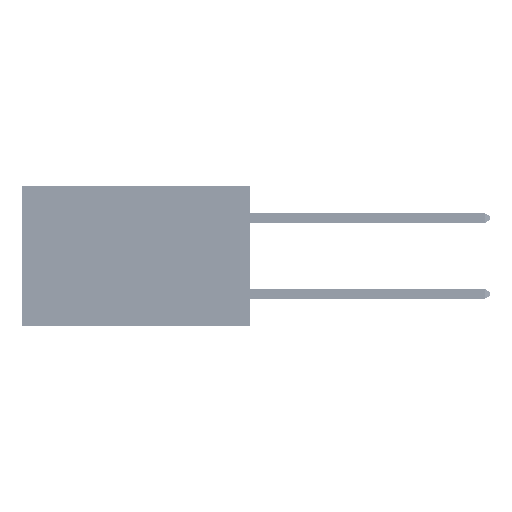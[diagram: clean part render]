
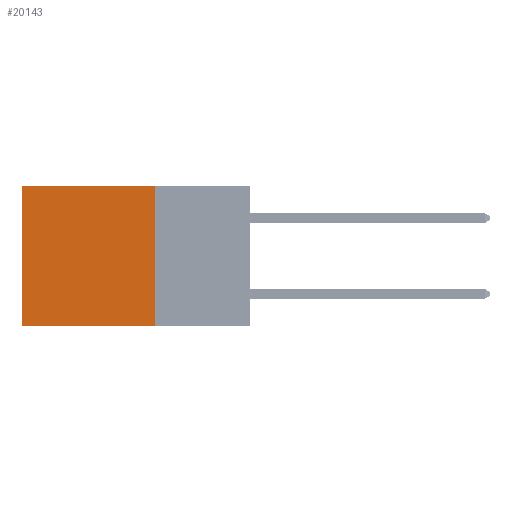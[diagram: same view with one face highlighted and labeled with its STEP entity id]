
A CAD part, left-side view. The second image highlights one B-rep face of the part: STEP entity #20143.
In plain terms, the highlighted planar face has unit normal (-1, 0, 0).
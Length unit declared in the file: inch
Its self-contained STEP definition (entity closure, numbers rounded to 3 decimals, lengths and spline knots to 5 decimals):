
#1675 = ORIENTED_EDGE ( 'NONE', *, *, #20244, .F. ) ;
#1763 = CARTESIAN_POINT ( 'NONE',  ( 0.2875, 0.25, 0. ) ) ;
#2349 = CARTESIAN_POINT ( 'NONE',  ( 0.2875, 0.25, -0.37 ) ) ;
#2363 = EDGE_CURVE ( 'NONE', #16972, #2997, #5981, .T. ) ;
#2503 = VECTOR ( 'NONE', #47408, 39.37008 ) ;
#2991 = VECTOR ( 'NONE', #42047, 39.37008 ) ;
#2997 = VERTEX_POINT ( 'NONE', #21439 ) ;
#5364 = DIRECTION ( 'NONE',  ( 0., 1., 0. ) ) ;
#5388 = EDGE_CURVE ( 'NONE', #8325, #2997, #25424, .T. ) ;
#5735 = CARTESIAN_POINT ( 'NONE',  ( 0.2875, 0.25, 0. ) ) ;
#5981 = LINE ( 'NONE', #14058, #2503 ) ;
#6455 = LINE ( 'NONE', #1763, #2991 ) ;
#6646 = VECTOR ( 'NONE', #5364, 39.37008 ) ;
#8325 = VERTEX_POINT ( 'NONE', #47046 ) ;
#9017 = VERTEX_POINT ( 'NONE', #5735 ) ;
#9226 = CARTESIAN_POINT ( 'NONE',  ( 0.2875, 0.25, 0. ) ) ;
#10490 = DIRECTION ( 'NONE',  ( 0., 0., -1. ) ) ;
#12920 = DIRECTION ( 'NONE',  ( 0., 0., -1. ) ) ;
#13207 = AXIS2_PLACEMENT_3D ( 'NONE', #38654, #34920, #12920 ) ;
#14058 = CARTESIAN_POINT ( 'NONE',  ( 0.2875, 0.25, -0.37 ) ) ;
#16972 = VERTEX_POINT ( 'NONE', #2349 ) ;
#20143 = ADVANCED_FACE ( 'NONE', ( #24960 ), #38502, .F. ) ;
#20244 = EDGE_CURVE ( 'NONE', #9017, #16972, #6455, .T. ) ;
#20344 = ORIENTED_EDGE ( 'NONE', *, *, #5388, .T. ) ;
#21439 = CARTESIAN_POINT ( 'NONE',  ( 0.2875, 0.6, -0.37 ) ) ;
#23466 = ORIENTED_EDGE ( 'NONE', *, *, #2363, .F. ) ;
#23699 = VECTOR ( 'NONE', #10490, 39.37008 ) ;
#24960 = FACE_OUTER_BOUND ( 'NONE', #39020, .T. ) ;
#25379 = EDGE_CURVE ( 'NONE', #9017, #8325, #39043, .T. ) ;
#25424 = LINE ( 'NONE', #32612, #23699 ) ;
#32612 = CARTESIAN_POINT ( 'NONE',  ( 0.2875, 0.6, 0. ) ) ;
#34920 = DIRECTION ( 'NONE',  ( 1., 0., 0. ) ) ;
#38502 = PLANE ( 'NONE',  #13207 ) ;
#38654 = CARTESIAN_POINT ( 'NONE',  ( 0.2875, 0.25, 0. ) ) ;
#39020 = EDGE_LOOP ( 'NONE', ( #20344, #23466, #1675, #45580 ) ) ;
#39043 = LINE ( 'NONE', #9226, #6646 ) ;
#42047 = DIRECTION ( 'NONE',  ( 0., 0., -1. ) ) ;
#45580 = ORIENTED_EDGE ( 'NONE', *, *, #25379, .T. ) ;
#47046 = CARTESIAN_POINT ( 'NONE',  ( 0.2875, 0.6, 0. ) ) ;
#47408 = DIRECTION ( 'NONE',  ( 0., 1., 0. ) ) ;
